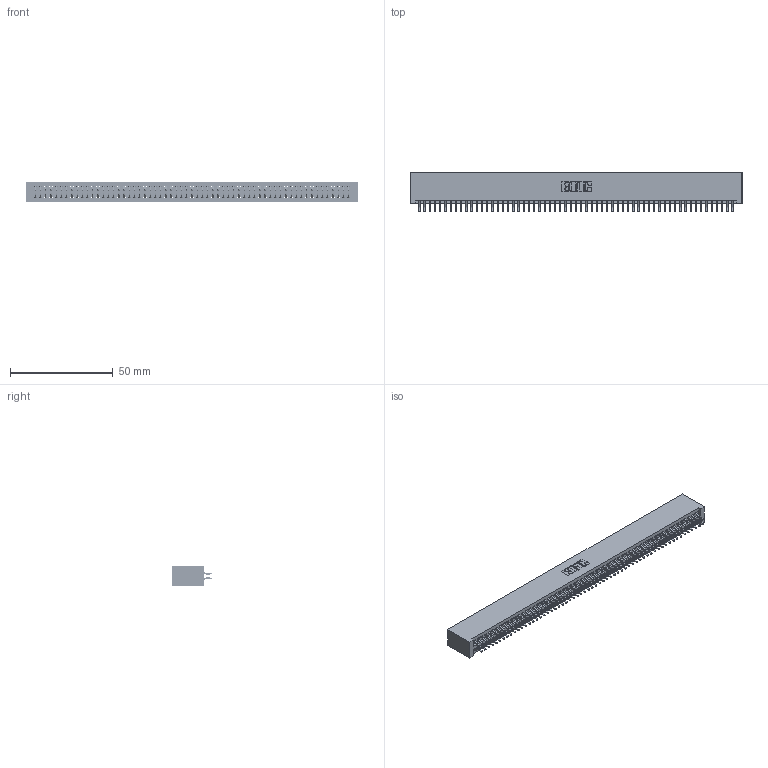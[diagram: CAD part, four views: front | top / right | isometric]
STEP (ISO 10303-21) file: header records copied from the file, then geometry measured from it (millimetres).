
FILE_DESCRIPTION (( 'STEP AP203' ), '1' );
FILE_NAME ('395-122-556-201.STEP', '2019-10-28T08:58:14', ( '' ), ( '' ), 'SwSTEP 2.0', 'SolidWorks 2016', '' );
FILE_SCHEMA (( 'CONFIG_CONTROL_DESIGN' ));
Length unit declared in the file: inch
Products named in the file (3): 345 Part_No Mounting Lugs; 345-292-001_556 Tail; 395-122-556-201
Assembly tree (123 placements, depth 2):
  395-122-556-201
    345 Part_No Mounting Lugs
    345-292-001_556 Tail  x122
Bounding box: 161.54 x 19.24 x 9.4 mm (x, y, z)
Volume: 16480 mm3; surface area: 24924.7 mm2
Topology: 123 solids, 123 shells, 6950 faces, 20691 edges, 13630 vertices
Faces by surface type: plane 4590, cylinder 2360
Entity records: 45247 total; most frequent: CARTESIAN_POINT 7580, ORIENTED_EDGE 7502, DIRECTION 6643, EDGE_CURVE 3751, VECTOR 3375, LINE 3375, VERTEX_POINT 2498, AXIS2_PLACEMENT_3D 1634
